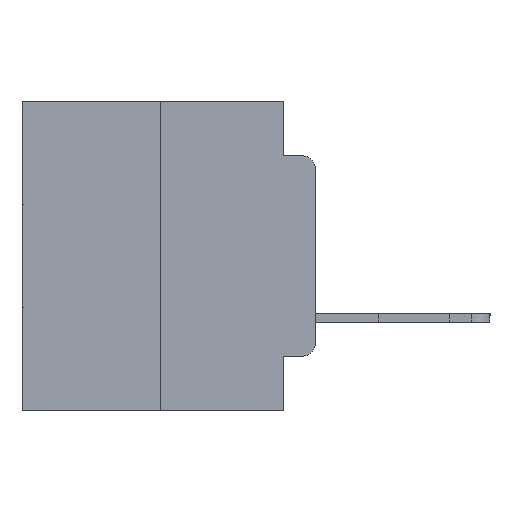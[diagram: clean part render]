
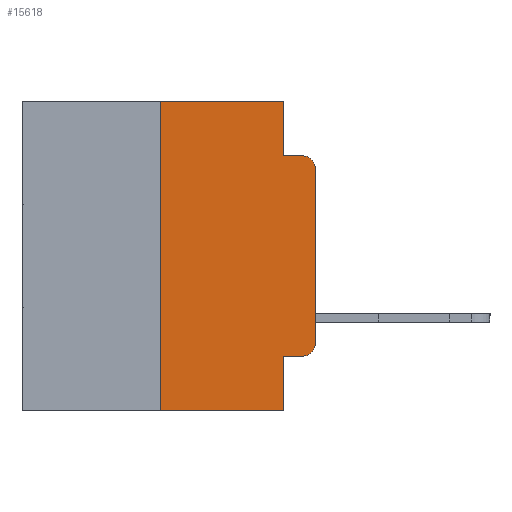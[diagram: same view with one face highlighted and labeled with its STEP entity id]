
A CAD part, left-side view. The second image highlights one B-rep face of the part: STEP entity #15618.
In plain terms, the highlighted planar face has unit normal (-1, 0, 0).
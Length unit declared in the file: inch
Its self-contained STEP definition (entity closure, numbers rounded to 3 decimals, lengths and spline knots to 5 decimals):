
#144 = ORIENTED_EDGE ( 'NONE', *, *, #17548, .F. ) ;
#337 = VECTOR ( 'NONE', #18415, 39.37008 ) ;
#521 = EDGE_CURVE ( 'NONE', #10942, #11726, #2342, .T. ) ;
#1272 = ORIENTED_EDGE ( 'NONE', *, *, #521, .T. ) ;
#1913 = DIRECTION ( 'NONE',  ( 0., 0., -1. ) ) ;
#2110 = ORIENTED_EDGE ( 'NONE', *, *, #7876, .T. ) ;
#2342 = LINE ( 'NONE', #25580, #25984 ) ;
#2661 = ORIENTED_EDGE ( 'NONE', *, *, #27244, .T. ) ;
#3506 = DIRECTION ( 'NONE',  ( 0., 0., 1. ) ) ;
#4157 = CIRCLE ( 'NONE', #6977, 0.02 ) ;
#4489 = LINE ( 'NONE', #8479, #9683 ) ;
#4633 = CARTESIAN_POINT ( 'NONE',  ( 0., 0.02, -0.0885 ) ) ;
#4864 = VECTOR ( 'NONE', #10910, 39.37008 ) ;
#5194 = ORIENTED_EDGE ( 'NONE', *, *, #12353, .F. ) ;
#5412 = EDGE_LOOP ( 'NONE', ( #1272, #2661, #5428, #144, #15766, #7614, #2110, #5194, #8545, #20086 ) ) ;
#5428 = ORIENTED_EDGE ( 'NONE', *, *, #18942, .F. ) ;
#5439 = VERTEX_POINT ( 'NONE', #13346 ) ;
#5908 = EDGE_CURVE ( 'NONE', #14392, #10942, #4157, .T. ) ;
#6257 = CARTESIAN_POINT ( 'NONE',  ( 0., 0.25, 0. ) ) ;
#6977 = AXIS2_PLACEMENT_3D ( 'NONE', #9971, #24792, #12179 ) ;
#7135 = VECTOR ( 'NONE', #27672, 39.37008 ) ;
#7433 = CARTESIAN_POINT ( 'NONE',  ( 0., 0.02, -0.4115 ) ) ;
#7614 = ORIENTED_EDGE ( 'NONE', *, *, #22287, .F. ) ;
#7876 = EDGE_CURVE ( 'NONE', #24763, #15770, #27707, .T. ) ;
#7894 = CARTESIAN_POINT ( 'NONE',  ( 0., 0.25, -0.5 ) ) ;
#8479 = CARTESIAN_POINT ( 'NONE',  ( 0., 0.051, 0. ) ) ;
#8545 = ORIENTED_EDGE ( 'NONE', *, *, #14689, .T. ) ;
#9683 = VECTOR ( 'NONE', #23419, 39.37008 ) ;
#9845 = DIRECTION ( 'NONE',  ( 0., -1., 0. ) ) ;
#9971 = CARTESIAN_POINT ( 'NONE',  ( 0., 0.02, -0.3915 ) ) ;
#10452 = VECTOR ( 'NONE', #3506, 39.37008 ) ;
#10718 = DIRECTION ( 'NONE',  ( 0., -1., 0. ) ) ;
#10839 = CARTESIAN_POINT ( 'NONE',  ( 0., 0.473, 0. ) ) ;
#10910 = DIRECTION ( 'NONE',  ( 0., -1., 0. ) ) ;
#10942 = VERTEX_POINT ( 'NONE', #27919 ) ;
#11204 = CARTESIAN_POINT ( 'NONE',  ( 0., 0.051, 0. ) ) ;
#11726 = VERTEX_POINT ( 'NONE', #19985 ) ;
#12179 = DIRECTION ( 'NONE',  ( 0., 0., -1. ) ) ;
#12353 = EDGE_CURVE ( 'NONE', #5439, #15770, #18146, .T. ) ;
#12590 = LINE ( 'NONE', #24674, #18259 ) ;
#12595 = VERTEX_POINT ( 'NONE', #11204 ) ;
#12606 = VERTEX_POINT ( 'NONE', #4633 ) ;
#13046 = DIRECTION ( 'NONE',  ( 0., 0., 1. ) ) ;
#13152 = PLANE ( 'NONE',  #22210 ) ;
#13330 = VERTEX_POINT ( 'NONE', #6257 ) ;
#13346 = CARTESIAN_POINT ( 'NONE',  ( 0., 0.051, -0.4115 ) ) ;
#13391 = DIRECTION ( 'NONE',  ( -1., 0., 0. ) ) ;
#13677 = LINE ( 'NONE', #17373, #7135 ) ;
#14392 = VERTEX_POINT ( 'NONE', #7433 ) ;
#14511 = CARTESIAN_POINT ( 'NONE',  ( 0., 0.25, 0. ) ) ;
#14689 = EDGE_CURVE ( 'NONE', #5439, #14392, #20745, .T. ) ;
#14890 = VERTEX_POINT ( 'NONE', #23213 ) ;
#15255 = DIRECTION ( 'NONE',  ( 1., 0., 0. ) ) ;
#15618 = ADVANCED_FACE ( 'NONE', ( #18706 ), #13152, .F. ) ;
#15766 = ORIENTED_EDGE ( 'NONE', *, *, #20344, .F. ) ;
#15770 = VERTEX_POINT ( 'NONE', #20068 ) ;
#15894 = AXIS2_PLACEMENT_3D ( 'NONE', #25915, #13391, #27954 ) ;
#17373 = CARTESIAN_POINT ( 'NONE',  ( 0., 0.051, -0.0885 ) ) ;
#17548 = EDGE_CURVE ( 'NONE', #12595, #14890, #4489, .T. ) ;
#18146 = LINE ( 'NONE', #20540, #337 ) ;
#18259 = VECTOR ( 'NONE', #9845, 39.37008 ) ;
#18415 = DIRECTION ( 'NONE',  ( 0., 0., -1. ) ) ;
#18706 = FACE_OUTER_BOUND ( 'NONE', #5412, .T. ) ;
#18942 = EDGE_CURVE ( 'NONE', #14890, #12606, #13677, .T. ) ;
#19985 = CARTESIAN_POINT ( 'NONE',  ( 0., 0., -0.1085 ) ) ;
#20068 = CARTESIAN_POINT ( 'NONE',  ( 0., 0.051, -0.5 ) ) ;
#20086 = ORIENTED_EDGE ( 'NONE', *, *, #5908, .T. ) ;
#20344 = EDGE_CURVE ( 'NONE', #13330, #12595, #12590, .T. ) ;
#20540 = CARTESIAN_POINT ( 'NONE',  ( 0., 0.051, 0. ) ) ;
#20745 = LINE ( 'NONE', #25662, #4864 ) ;
#22210 = AXIS2_PLACEMENT_3D ( 'NONE', #10839, #15255, #1913 ) ;
#22287 = EDGE_CURVE ( 'NONE', #24763, #13330, #27218, .T. ) ;
#23213 = CARTESIAN_POINT ( 'NONE',  ( 0., 0.051, -0.0885 ) ) ;
#23419 = DIRECTION ( 'NONE',  ( 0., 0., -1. ) ) ;
#24674 = CARTESIAN_POINT ( 'NONE',  ( 0., 0.473, 0. ) ) ;
#24763 = VERTEX_POINT ( 'NONE', #7894 ) ;
#24792 = DIRECTION ( 'NONE',  ( -1., 0., 0. ) ) ;
#25397 = CARTESIAN_POINT ( 'NONE',  ( 0., 0.473, -0.5 ) ) ;
#25580 = CARTESIAN_POINT ( 'NONE',  ( 0., 0., 0. ) ) ;
#25662 = CARTESIAN_POINT ( 'NONE',  ( 0., 0.051, -0.4115 ) ) ;
#25915 = CARTESIAN_POINT ( 'NONE',  ( 0., 0.02, -0.1085 ) ) ;
#25984 = VECTOR ( 'NONE', #13046, 39.37008 ) ;
#26440 = VECTOR ( 'NONE', #10718, 39.37008 ) ;
#26755 = CIRCLE ( 'NONE', #15894, 0.02 ) ;
#27218 = LINE ( 'NONE', #14511, #10452 ) ;
#27244 = EDGE_CURVE ( 'NONE', #11726, #12606, #26755, .T. ) ;
#27672 = DIRECTION ( 'NONE',  ( 0., -1., 0. ) ) ;
#27707 = LINE ( 'NONE', #25397, #26440 ) ;
#27919 = CARTESIAN_POINT ( 'NONE',  ( 0., 0., -0.3915 ) ) ;
#27954 = DIRECTION ( 'NONE',  ( 0., 0., -1. ) ) ;
